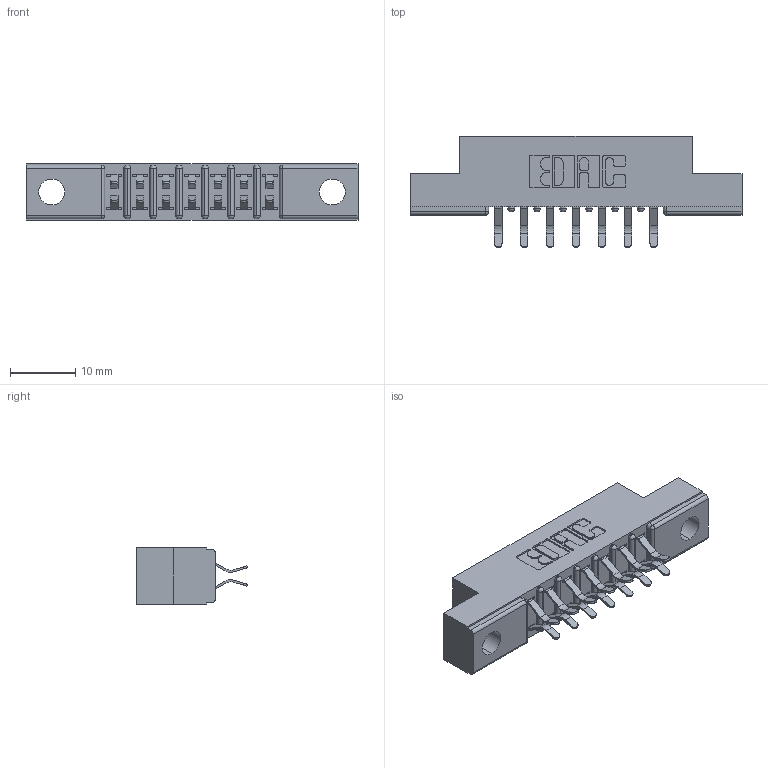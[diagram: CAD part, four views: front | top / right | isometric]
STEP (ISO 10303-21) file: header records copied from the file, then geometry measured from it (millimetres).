
FILE_DESCRIPTION (( 'STEP AP203' ), '1' );
FILE_NAME ('357-014-556-204.STEP', '2019-09-17T18:43:56', ( '' ), ( '' ), 'SwSTEP 2.0', 'SolidWorks 2016', '' );
FILE_SCHEMA (( 'CONFIG_CONTROL_DESIGN' ));
Length unit declared in the file: inch
Products named in the file (3): 357-014-556-204; 307-290-001_556; 307 Part_.156 Dia Mounting Holes
Assembly tree (15 placements, depth 2):
  357-014-556-204
    307 Part_.156 Dia Mounting Holes
    307-290-001_556  x14
Bounding box: 50.75 x 16.97 x 8.71 mm (x, y, z)
Volume: 3212.7 mm3; surface area: 4766.7 mm2
Topology: 15 solids, 15 shells, 840 faces, 2347 edges, 1522 vertices
Faces by surface type: plane 546, cylinder 278, sphere 16
Entity records: 11062 total; most frequent: CARTESIAN_POINT 1825, ORIENTED_EDGE 1802, DIRECTION 1795, EDGE_CURVE 901, VECTOR 683, LINE 683, VERTEX_POINT 586, AXIS2_PLACEMENT_3D 556
